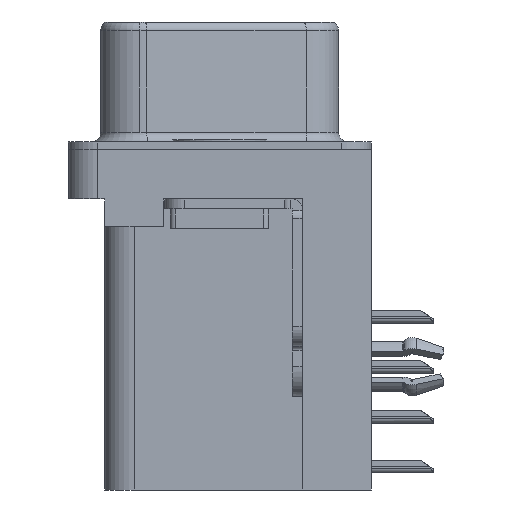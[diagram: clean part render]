
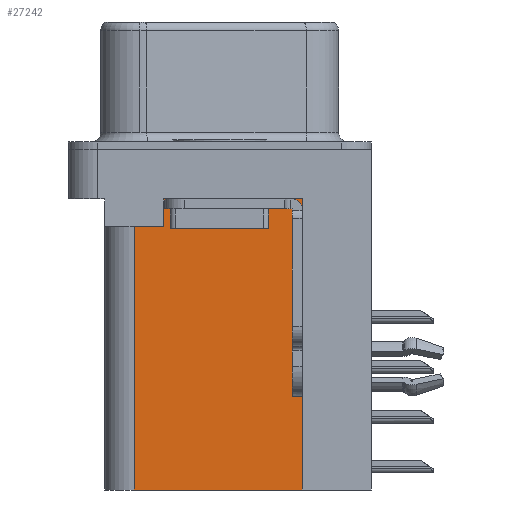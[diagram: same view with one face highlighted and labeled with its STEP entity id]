
A CAD part, left-side view. The second image highlights one B-rep face of the part: STEP entity #27242.
In plain terms, the highlighted planar face has unit normal (-1, 0, 0).
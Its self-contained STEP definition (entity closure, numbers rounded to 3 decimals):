
#917 = CARTESIAN_POINT ( 'NONE',  ( 3.75, 2.85, -3.9 ) ) ;
#992 = DIRECTION ( 'NONE',  ( 0., 0., 1. ) ) ;
#2089 = EDGE_LOOP ( 'NONE', ( #21287, #21496, #35466, #11131, #2478, #25494 ) ) ;
#2478 = ORIENTED_EDGE ( 'NONE', *, *, #13966, .F. ) ;
#2836 = LINE ( 'NONE', #13657, #27015 ) ;
#5754 = CARTESIAN_POINT ( 'NONE',  ( 3.75, -4.2, -17.3 ) ) ;
#8157 = AXIS2_PLACEMENT_3D ( 'NONE', #34400, #28235, #9418 ) ;
#8463 = LINE ( 'NONE', #917, #24210 ) ;
#8544 = CARTESIAN_POINT ( 'NONE',  ( 3.75, 2.85, -3.9 ) ) ;
#9418 = DIRECTION ( 'NONE',  ( 0., 1., 0. ) ) ;
#10021 = VECTOR ( 'NONE', #21922, 1000. ) ;
#10803 = LINE ( 'NONE', #23233, #26509 ) ;
#11131 = ORIENTED_EDGE ( 'NONE', *, *, #39225, .F. ) ;
#12440 = VECTOR ( 'NONE', #37191, 1000. ) ;
#13657 = CARTESIAN_POINT ( 'NONE',  ( 3.75, -4.2, -2.5 ) ) ;
#13966 = EDGE_CURVE ( 'NONE', #33331, #39360, #21404, .T. ) ;
#14105 = VERTEX_POINT ( 'NONE', #16083 ) ;
#15141 = CARTESIAN_POINT ( 'NONE',  ( 3.75, -4.2, -17.3 ) ) ;
#15238 = CARTESIAN_POINT ( 'NONE',  ( 3.75, 4.35, -17.3 ) ) ;
#15375 = CARTESIAN_POINT ( 'NONE',  ( 3.75, 4.35, -3.9 ) ) ;
#16072 = EDGE_CURVE ( 'NONE', #14105, #16285, #8463, .T. ) ;
#16083 = CARTESIAN_POINT ( 'NONE',  ( 3.75, 2.85, -2.5 ) ) ;
#16285 = VERTEX_POINT ( 'NONE', #8544 ) ;
#16862 = CARTESIAN_POINT ( 'NONE',  ( 3.75, -4.2, -2.5 ) ) ;
#16879 = DIRECTION ( 'NONE',  ( 0., 0., -1. ) ) ;
#17761 = VERTEX_POINT ( 'NONE', #15375 ) ;
#18754 = CARTESIAN_POINT ( 'NONE',  ( 3.75, 0., -3.9 ) ) ;
#19395 = LINE ( 'NONE', #18754, #10021 ) ;
#21287 = ORIENTED_EDGE ( 'NONE', *, *, #33098, .T. ) ;
#21404 = LINE ( 'NONE', #15141, #30684 ) ;
#21496 = ORIENTED_EDGE ( 'NONE', *, *, #16072, .T. ) ;
#21922 = DIRECTION ( 'NONE',  ( 0., 1., 0. ) ) ;
#21964 = PLANE ( 'NONE',  #8157 ) ;
#22127 = FACE_OUTER_BOUND ( 'NONE', #2089, .T. ) ;
#23233 = CARTESIAN_POINT ( 'NONE',  ( 3.75, -4.2, -17.3 ) ) ;
#24189 = EDGE_CURVE ( 'NONE', #16285, #17761, #19395, .T. ) ;
#24210 = VECTOR ( 'NONE', #16879, 1000. ) ;
#25196 = CARTESIAN_POINT ( 'NONE',  ( 3.75, 4.35, -17.3 ) ) ;
#25494 = ORIENTED_EDGE ( 'NONE', *, *, #33604, .T. ) ;
#26509 = VECTOR ( 'NONE', #992, 1000. ) ;
#27015 = VECTOR ( 'NONE', #29391, 1000. ) ;
#27242 = ADVANCED_FACE ( 'NONE', ( #22127 ), #21964, .F. ) ;
#28235 = DIRECTION ( 'NONE',  ( 1., 0., 0. ) ) ;
#29391 = DIRECTION ( 'NONE',  ( 0., 1., 0. ) ) ;
#30684 = VECTOR ( 'NONE', #34007, 1000. ) ;
#31092 = LINE ( 'NONE', #15238, #12440 ) ;
#33098 = EDGE_CURVE ( 'NONE', #39573, #14105, #2836, .T. ) ;
#33331 = VERTEX_POINT ( 'NONE', #5754 ) ;
#33604 = EDGE_CURVE ( 'NONE', #33331, #39573, #10803, .T. ) ;
#34007 = DIRECTION ( 'NONE',  ( 0., 1., 0. ) ) ;
#34400 = CARTESIAN_POINT ( 'NONE',  ( 3.75, -4.2, -17.3 ) ) ;
#35466 = ORIENTED_EDGE ( 'NONE', *, *, #24189, .T. ) ;
#37191 = DIRECTION ( 'NONE',  ( 0., 0., 1. ) ) ;
#39225 = EDGE_CURVE ( 'NONE', #39360, #17761, #31092, .T. ) ;
#39360 = VERTEX_POINT ( 'NONE', #25196 ) ;
#39573 = VERTEX_POINT ( 'NONE', #16862 ) ;
